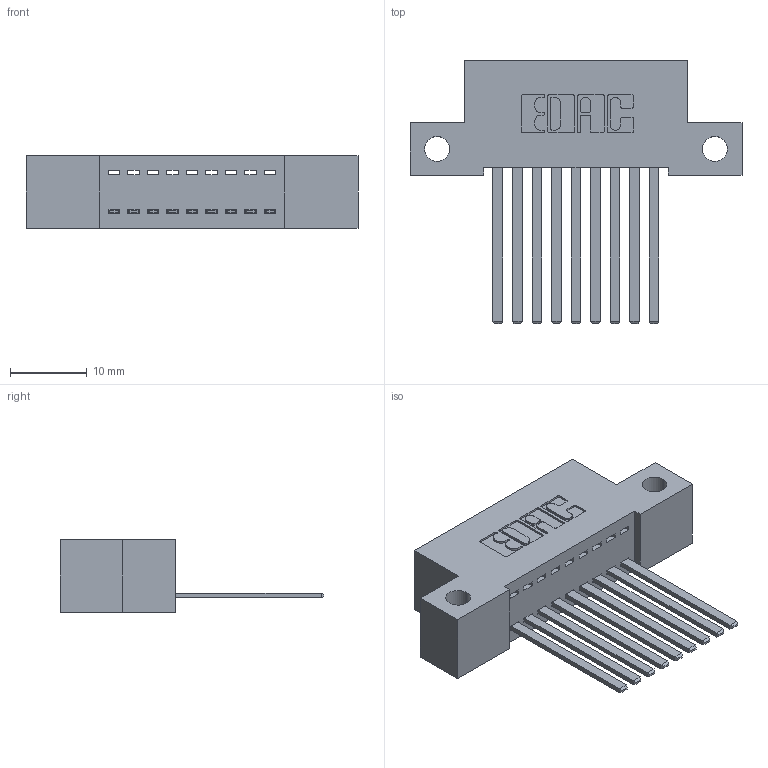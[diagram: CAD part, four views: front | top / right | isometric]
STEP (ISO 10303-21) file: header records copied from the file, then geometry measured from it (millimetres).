
FILE_DESCRIPTION (( 'STEP AP203' ), '1' );
FILE_NAME ('342-009-544-112.STEP', '2019-10-01T13:35:17', ( '' ), ( '' ), 'SwSTEP 2.0', 'SolidWorks 2016', '' );
FILE_SCHEMA (( 'CONFIG_CONTROL_DESIGN' ));
Length unit declared in the file: inch
Products named in the file (3): 342 Part_Side Mount; 345-292-001_345-293-144; 342-009-544-112
Assembly tree (10 placements, depth 2):
  342-009-544-112
    342 Part_Side Mount
    345-292-001_345-293-144  x9
Bounding box: 43.18 x 34.3 x 9.4 mm (x, y, z)
Volume: 3694.8 mm3; surface area: 4943 mm2
Topology: 10 solids, 10 shells, 578 faces, 1721 edges, 1134 vertices
Faces by surface type: plane 408, cylinder 170
Entity records: 9457 total; most frequent: CARTESIAN_POINT 1641, ORIENTED_EDGE 1586, DIRECTION 1447, EDGE_CURVE 793, LINE 669, VECTOR 669, VERTEX_POINT 526, AXIS2_PLACEMENT_3D 389
